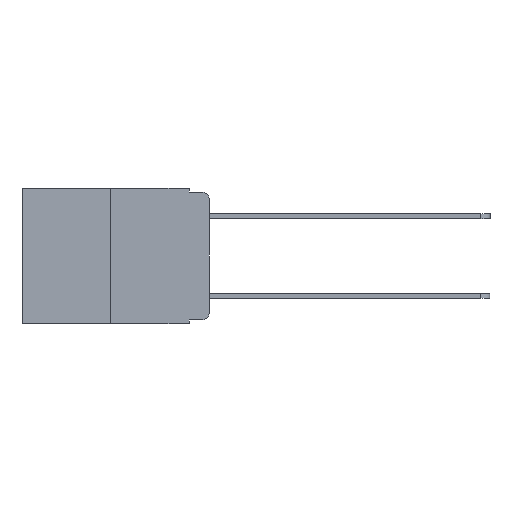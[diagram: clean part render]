
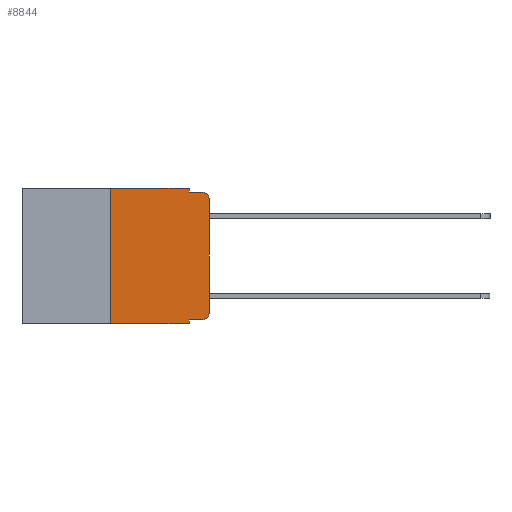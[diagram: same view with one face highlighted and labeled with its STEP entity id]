
A CAD part, left-side view. The second image highlights one B-rep face of the part: STEP entity #8844.
In plain terms, the highlighted planar face has unit normal (-1, 0, 0).
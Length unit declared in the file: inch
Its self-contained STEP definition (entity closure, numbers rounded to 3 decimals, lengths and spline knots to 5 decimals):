
#22 = VERTEX_POINT ( 'NONE', #7783 ) ;
#66 = CARTESIAN_POINT ( 'NONE',  ( 0., 0.051, -0.01 ) ) ;
#107 = PLANE ( 'NONE',  #2587 ) ;
#120 = DIRECTION ( 'NONE',  ( 0., -1., 0. ) ) ;
#249 = ORIENTED_EDGE ( 'NONE', *, *, #8034, .T. ) ;
#355 = VERTEX_POINT ( 'NONE', #6992 ) ;
#397 = FACE_OUTER_BOUND ( 'NONE', #6351, .T. ) ;
#409 = VERTEX_POINT ( 'NONE', #4214 ) ;
#515 = ORIENTED_EDGE ( 'NONE', *, *, #2211, .T. ) ;
#562 = DIRECTION ( 'NONE',  ( -1., 0., 0. ) ) ;
#751 = EDGE_CURVE ( 'NONE', #3473, #409, #4125, .T. ) ;
#1003 = AXIS2_PLACEMENT_3D ( 'NONE', #5338, #562, #6122 ) ;
#1349 = CARTESIAN_POINT ( 'NONE',  ( 0., 0.473, 0. ) ) ;
#1464 = DIRECTION ( 'NONE',  ( 0., 0., 1. ) ) ;
#1559 = EDGE_CURVE ( 'NONE', #22, #2710, #4608, .T. ) ;
#1758 = CARTESIAN_POINT ( 'NONE',  ( 0., 0.473, 0. ) ) ;
#1861 = VECTOR ( 'NONE', #120, 39.37008 ) ;
#1882 = LINE ( 'NONE', #4393, #9607 ) ;
#1962 = CARTESIAN_POINT ( 'NONE',  ( 0., 0., 0. ) ) ;
#2010 = VECTOR ( 'NONE', #5508, 39.37008 ) ;
#2163 = VERTEX_POINT ( 'NONE', #8547 ) ;
#2211 = EDGE_CURVE ( 'NONE', #6668, #4318, #2365, .T. ) ;
#2237 = LINE ( 'NONE', #9777, #9680 ) ;
#2248 = ORIENTED_EDGE ( 'NONE', *, *, #6453, .T. ) ;
#2341 = CIRCLE ( 'NONE', #1003, 0.02 ) ;
#2365 = LINE ( 'NONE', #1962, #5793 ) ;
#2406 = EDGE_CURVE ( 'NONE', #2163, #22, #2237, .T. ) ;
#2587 = AXIS2_PLACEMENT_3D ( 'NONE', #1758, #8599, #4166 ) ;
#2710 = VERTEX_POINT ( 'NONE', #6575 ) ;
#3107 = ORIENTED_EDGE ( 'NONE', *, *, #2406, .F. ) ;
#3221 = DIRECTION ( 'NONE',  ( 0., -1., 0. ) ) ;
#3473 = VERTEX_POINT ( 'NONE', #4384 ) ;
#3692 = DIRECTION ( 'NONE',  ( 0., 0., -1. ) ) ;
#3732 = ORIENTED_EDGE ( 'NONE', *, *, #7225, .T. ) ;
#3758 = DIRECTION ( 'NONE',  ( 0., 0., 1. ) ) ;
#3765 = ORIENTED_EDGE ( 'NONE', *, *, #751, .F. ) ;
#3942 = DIRECTION ( 'NONE',  ( 0., -1., 0. ) ) ;
#3992 = LINE ( 'NONE', #5703, #1861 ) ;
#4125 = LINE ( 'NONE', #4171, #2010 ) ;
#4166 = DIRECTION ( 'NONE',  ( 0., 0., -1. ) ) ;
#4171 = CARTESIAN_POINT ( 'NONE',  ( 0., 0.051, 0. ) ) ;
#4214 = CARTESIAN_POINT ( 'NONE',  ( 0., 0.051, -0.343 ) ) ;
#4318 = VERTEX_POINT ( 'NONE', #4915 ) ;
#4329 = CARTESIAN_POINT ( 'NONE',  ( 0., 0.02, -0.313 ) ) ;
#4384 = CARTESIAN_POINT ( 'NONE',  ( 0., 0.051, -0.333 ) ) ;
#4393 = CARTESIAN_POINT ( 'NONE',  ( 0., 0.051, 0. ) ) ;
#4552 = VECTOR ( 'NONE', #3942, 39.37008 ) ;
#4608 = LINE ( 'NONE', #1349, #6394 ) ;
#4887 = DIRECTION ( 'NONE',  ( 0., -1., 0. ) ) ;
#4915 = CARTESIAN_POINT ( 'NONE',  ( 0., 0., -0.03 ) ) ;
#5116 = DIRECTION ( 'NONE',  ( 0., 0., -1. ) ) ;
#5338 = CARTESIAN_POINT ( 'NONE',  ( 0., 0.02, -0.03 ) ) ;
#5343 = ORIENTED_EDGE ( 'NONE', *, *, #8645, .T. ) ;
#5508 = DIRECTION ( 'NONE',  ( 0., 0., -1. ) ) ;
#5552 = EDGE_CURVE ( 'NONE', #2710, #355, #1882, .T. ) ;
#5666 = VECTOR ( 'NONE', #4887, 39.37008 ) ;
#5703 = CARTESIAN_POINT ( 'NONE',  ( 0., 0.473, -0.343 ) ) ;
#5793 = VECTOR ( 'NONE', #1464, 39.37008 ) ;
#5908 = LINE ( 'NONE', #66, #5666 ) ;
#6006 = CARTESIAN_POINT ( 'NONE',  ( 0., 0.02, -0.01 ) ) ;
#6122 = DIRECTION ( 'NONE',  ( 0., 0., -1. ) ) ;
#6347 = LINE ( 'NONE', #8402, #4552 ) ;
#6351 = EDGE_LOOP ( 'NONE', ( #515, #249, #6393, #8694, #7662, #3107, #2248, #3765, #5343, #3732 ) ) ;
#6393 = ORIENTED_EDGE ( 'NONE', *, *, #7038, .F. ) ;
#6394 = VECTOR ( 'NONE', #3221, 39.37008 ) ;
#6453 = EDGE_CURVE ( 'NONE', #2163, #409, #3992, .T. ) ;
#6575 = CARTESIAN_POINT ( 'NONE',  ( 0., 0.051, 0. ) ) ;
#6668 = VERTEX_POINT ( 'NONE', #8139 ) ;
#6709 = VERTEX_POINT ( 'NONE', #6006 ) ;
#6992 = CARTESIAN_POINT ( 'NONE',  ( 0., 0.051, -0.01 ) ) ;
#7038 = EDGE_CURVE ( 'NONE', #355, #6709, #5908, .T. ) ;
#7225 = EDGE_CURVE ( 'NONE', #9651, #6668, #9783, .T. ) ;
#7662 = ORIENTED_EDGE ( 'NONE', *, *, #1559, .F. ) ;
#7783 = CARTESIAN_POINT ( 'NONE',  ( 0., 0.25, 0. ) ) ;
#8034 = EDGE_CURVE ( 'NONE', #4318, #6709, #2341, .T. ) ;
#8139 = CARTESIAN_POINT ( 'NONE',  ( 0., 0., -0.313 ) ) ;
#8402 = CARTESIAN_POINT ( 'NONE',  ( 0., 0.051, -0.333 ) ) ;
#8547 = CARTESIAN_POINT ( 'NONE',  ( 0., 0.25, -0.343 ) ) ;
#8599 = DIRECTION ( 'NONE',  ( 1., 0., 0. ) ) ;
#8645 = EDGE_CURVE ( 'NONE', #3473, #9651, #6347, .T. ) ;
#8694 = ORIENTED_EDGE ( 'NONE', *, *, #5552, .F. ) ;
#8844 = ADVANCED_FACE ( 'NONE', ( #397 ), #107, .F. ) ;
#8984 = CARTESIAN_POINT ( 'NONE',  ( 0., 0.02, -0.333 ) ) ;
#9442 = DIRECTION ( 'NONE',  ( -1., 0., 0. ) ) ;
#9552 = AXIS2_PLACEMENT_3D ( 'NONE', #4329, #9442, #5116 ) ;
#9607 = VECTOR ( 'NONE', #3692, 39.37008 ) ;
#9651 = VERTEX_POINT ( 'NONE', #8984 ) ;
#9680 = VECTOR ( 'NONE', #3758, 39.37008 ) ;
#9777 = CARTESIAN_POINT ( 'NONE',  ( 0., 0.25, 0. ) ) ;
#9783 = CIRCLE ( 'NONE', #9552, 0.02 ) ;
